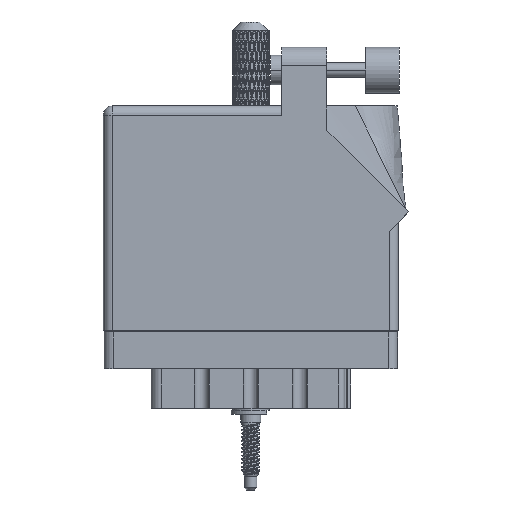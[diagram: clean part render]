
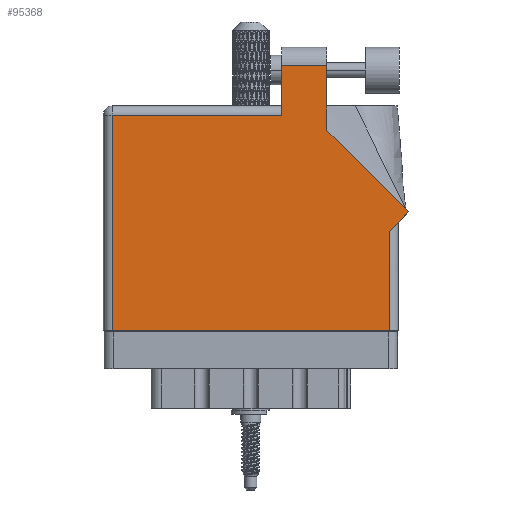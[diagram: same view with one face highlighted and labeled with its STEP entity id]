
A CAD part, front view. The second image highlights one B-rep face of the part: STEP entity #95368.
In plain terms, the highlighted face is planar.
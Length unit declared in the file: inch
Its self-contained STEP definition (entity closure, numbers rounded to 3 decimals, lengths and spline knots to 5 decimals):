
#721 = CARTESIAN_POINT ( 'NONE',  ( 1.948, 0.675, 0. ) ) ;
#1034 = VECTOR ( 'NONE', #97225, 39.37008 ) ;
#1722 = VERTEX_POINT ( 'NONE', #721 ) ;
#2205 = ORIENTED_EDGE ( 'NONE', *, *, #86111, .T. ) ;
#3090 = DIRECTION ( 'NONE',  ( 0., -1., 0. ) ) ;
#4298 = CARTESIAN_POINT ( 'NONE',  ( 1.948, 0., 0. ) ) ;
#5646 = LINE ( 'NONE', #105626, #46985 ) ;
#6546 = CARTESIAN_POINT ( 'NONE',  ( 1.524, 1.36442, 0. ) ) ;
#6810 = DIRECTION ( 'NONE',  ( 1., 0., 0. ) ) ;
#9564 = PLANE ( 'NONE',  #61883 ) ;
#11793 = ORIENTED_EDGE ( 'NONE', *, *, #49495, .T. ) ;
#13462 = ORIENTED_EDGE ( 'NONE', *, *, #16117, .T. ) ;
#14111 = CARTESIAN_POINT ( 'NONE',  ( 0.062, 1.468, 0. ) ) ;
#14427 = CARTESIAN_POINT ( 'NONE',  ( 0., 1.468, 0. ) ) ;
#15743 = DIRECTION ( 'NONE',  ( 0., 1., 0. ) ) ;
#16117 = EDGE_CURVE ( 'NONE', #87754, #58640, #33347, .T. ) ;
#17886 = CARTESIAN_POINT ( 'NONE',  ( 0., 1.53, 0. ) ) ;
#18369 = DIRECTION ( 'NONE',  ( 0.707, 0.707, 0. ) ) ;
#18647 = CARTESIAN_POINT ( 'NONE',  ( 1.217, 1.53, 0. ) ) ;
#20147 = CARTESIAN_POINT ( 'NONE',  ( 2.08071, 0.80771, 0. ) ) ;
#22889 = CARTESIAN_POINT ( 'NONE',  ( 0.062, 0., 0. ) ) ;
#24794 = VERTEX_POINT ( 'NONE', #20147 ) ;
#26631 = VECTOR ( 'NONE', #76943, 39.37008 ) ;
#31266 = ORIENTED_EDGE ( 'NONE', *, *, #42885, .T. ) ;
#32012 = CARTESIAN_POINT ( 'NONE',  ( 1.948, 0.737, 0. ) ) ;
#33066 = EDGE_LOOP ( 'NONE', ( #2205, #11793, #36468, #13462, #31266, #58650, #38982, #50650, #47517 ) ) ;
#33144 = CARTESIAN_POINT ( 'NONE',  ( 0.062, 0., 0. ) ) ;
#33347 = LINE ( 'NONE', #14427, #59127 ) ;
#35956 = VERTEX_POINT ( 'NONE', #4298 ) ;
#36468 = ORIENTED_EDGE ( 'NONE', *, *, #40583, .T. ) ;
#37012 = DIRECTION ( 'NONE',  ( 0., 0., -1. ) ) ;
#38098 = FACE_OUTER_BOUND ( 'NONE', #33066, .T. ) ;
#38982 = ORIENTED_EDGE ( 'NONE', *, *, #93307, .T. ) ;
#40583 = EDGE_CURVE ( 'NONE', #47899, #87754, #104155, .T. ) ;
#42885 = EDGE_CURVE ( 'NONE', #58640, #104389, #82413, .T. ) ;
#44112 = CARTESIAN_POINT ( 'NONE',  ( 2.08071, 0.80771, 0. ) ) ;
#45869 = CARTESIAN_POINT ( 'NONE',  ( 1.217, 1.805, 0. ) ) ;
#46985 = VECTOR ( 'NONE', #107082, 39.37008 ) ;
#47517 = ORIENTED_EDGE ( 'NONE', *, *, #76501, .T. ) ;
#47899 = VERTEX_POINT ( 'NONE', #87664 ) ;
#49495 = EDGE_CURVE ( 'NONE', #96831, #47899, #82955, .T. ) ;
#49838 = LINE ( 'NONE', #44112, #26631 ) ;
#50650 = ORIENTED_EDGE ( 'NONE', *, *, #103091, .T. ) ;
#52329 = VECTOR ( 'NONE', #18369, 39.37008 ) ;
#55631 = LINE ( 'NONE', #97780, #86580 ) ;
#58640 = VERTEX_POINT ( 'NONE', #14111 ) ;
#58650 = ORIENTED_EDGE ( 'NONE', *, *, #82658, .T. ) ;
#59127 = VECTOR ( 'NONE', #71101, 39.37008 ) ;
#60208 = CARTESIAN_POINT ( 'NONE',  ( 2.01, 0.737, 0. ) ) ;
#61883 = AXIS2_PLACEMENT_3D ( 'NONE', #17886, #37012, #102310 ) ;
#70764 = DIRECTION ( 'NONE',  ( -1., 0., 0. ) ) ;
#71101 = DIRECTION ( 'NONE',  ( -1., 0., 0. ) ) ;
#71849 = VECTOR ( 'NONE', #15743, 39.37008 ) ;
#76501 = EDGE_CURVE ( 'NONE', #24794, #76645, #49838, .T. ) ;
#76645 = VERTEX_POINT ( 'NONE', #6546 ) ;
#76678 = CARTESIAN_POINT ( 'NONE',  ( 1.524, 1.805, 0. ) ) ;
#76943 = DIRECTION ( 'NONE',  ( -0.707, 0.707, 0. ) ) ;
#79618 = VECTOR ( 'NONE', #3090, 39.37008 ) ;
#79787 = CARTESIAN_POINT ( 'NONE',  ( 1.217, 1.468, 0. ) ) ;
#82413 = LINE ( 'NONE', #22889, #1034 ) ;
#82658 = EDGE_CURVE ( 'NONE', #104389, #35956, #55631, .T. ) ;
#82955 = LINE ( 'NONE', #45869, #84172 ) ;
#84172 = VECTOR ( 'NONE', #70764, 39.37008 ) ;
#86009 = LINE ( 'NONE', #32012, #71849 ) ;
#86111 = EDGE_CURVE ( 'NONE', #76645, #96831, #5646, .T. ) ;
#86580 = VECTOR ( 'NONE', #6810, 39.37008 ) ;
#87664 = CARTESIAN_POINT ( 'NONE',  ( 1.217, 1.805, 0. ) ) ;
#87754 = VERTEX_POINT ( 'NONE', #79787 ) ;
#93307 = EDGE_CURVE ( 'NONE', #35956, #1722, #86009, .T. ) ;
#95368 = ADVANCED_FACE ( 'NONE', ( #38098 ), #9564, .F. ) ;
#96831 = VERTEX_POINT ( 'NONE', #76678 ) ;
#97225 = DIRECTION ( 'NONE',  ( 0., -1., 0. ) ) ;
#97780 = CARTESIAN_POINT ( 'NONE',  ( 0., 0., 0. ) ) ;
#98846 = LINE ( 'NONE', #60208, #52329 ) ;
#102310 = DIRECTION ( 'NONE',  ( -1., 0., 0. ) ) ;
#103091 = EDGE_CURVE ( 'NONE', #1722, #24794, #98846, .T. ) ;
#104155 = LINE ( 'NONE', #18647, #79618 ) ;
#104389 = VERTEX_POINT ( 'NONE', #33144 ) ;
#105626 = CARTESIAN_POINT ( 'NONE',  ( 1.524, 1.36442, 0. ) ) ;
#107082 = DIRECTION ( 'NONE',  ( 0., 1., 0. ) ) ;
